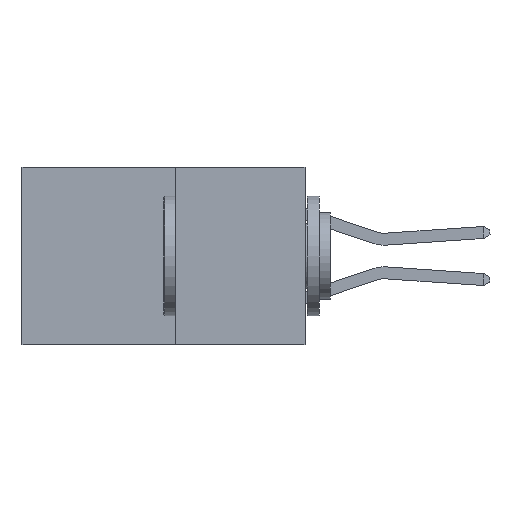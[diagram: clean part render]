
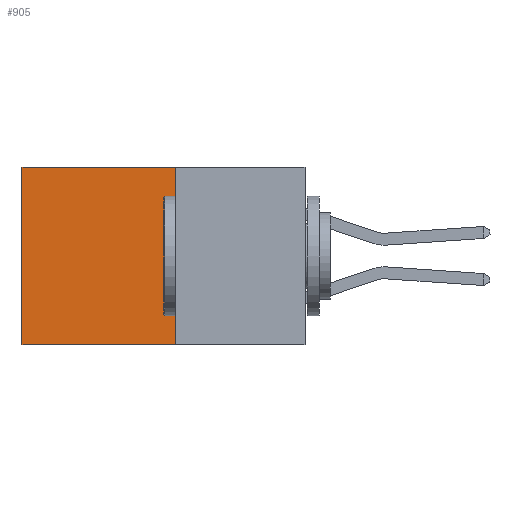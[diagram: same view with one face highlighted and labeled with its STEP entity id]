
A CAD part, left-side view. The second image highlights one B-rep face of the part: STEP entity #905.
In plain terms, the highlighted planar face has unit normal (-1, 0, 0).
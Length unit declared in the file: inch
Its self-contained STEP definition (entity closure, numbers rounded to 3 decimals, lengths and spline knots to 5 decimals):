
#81 = EDGE_CURVE ( 'NONE', #8730, #8609, #4554, .T. ) ;
#905 = ADVANCED_FACE ( 'NONE', ( #2821 ), #7786, .F. ) ;
#1059 = EDGE_CURVE ( 'NONE', #1190, #8609, #7743, .T. ) ;
#1190 = VERTEX_POINT ( 'NONE', #9414 ) ;
#2821 = FACE_OUTER_BOUND ( 'NONE', #2878, .T. ) ;
#2878 = EDGE_LOOP ( 'NONE', ( #4467, #7238, #5087, #5589 ) ) ;
#4222 = AXIS2_PLACEMENT_3D ( 'NONE', #8554, #8684, #8568 ) ;
#4467 = ORIENTED_EDGE ( 'NONE', *, *, #81, .T. ) ;
#4554 = LINE ( 'NONE', #9652, #10314 ) ;
#5087 = ORIENTED_EDGE ( 'NONE', *, *, #10065, .F. ) ;
#5205 = EDGE_CURVE ( 'NONE', #7248, #8730, #9862, .T. ) ;
#5479 = LINE ( 'NONE', #9789, #5730 ) ;
#5589 = ORIENTED_EDGE ( 'NONE', *, *, #5205, .T. ) ;
#5730 = VECTOR ( 'NONE', #10514, 39.37008 ) ;
#5748 = VECTOR ( 'NONE', #8367, 39.37008 ) ;
#5784 = CARTESIAN_POINT ( 'NONE',  ( 0.277, 0.59, -0.37 ) ) ;
#6378 = DIRECTION ( 'NONE',  ( 0., 0., -1. ) ) ;
#7238 = ORIENTED_EDGE ( 'NONE', *, *, #1059, .F. ) ;
#7248 = VERTEX_POINT ( 'NONE', #7903 ) ;
#7373 = CARTESIAN_POINT ( 'NONE',  ( 0.277, 0.59, 0. ) ) ;
#7743 = LINE ( 'NONE', #9202, #5748 ) ;
#7786 = PLANE ( 'NONE',  #4222 ) ;
#7889 = VECTOR ( 'NONE', #9340, 39.37008 ) ;
#7903 = CARTESIAN_POINT ( 'NONE',  ( 0.277, 0.27, 0. ) ) ;
#8367 = DIRECTION ( 'NONE',  ( 0., 1., 0. ) ) ;
#8554 = CARTESIAN_POINT ( 'NONE',  ( 0.277, 0.27, -0.37 ) ) ;
#8568 = DIRECTION ( 'NONE',  ( 0., 0., -1. ) ) ;
#8609 = VERTEX_POINT ( 'NONE', #5784 ) ;
#8684 = DIRECTION ( 'NONE',  ( 1., 0., 0. ) ) ;
#8730 = VERTEX_POINT ( 'NONE', #7373 ) ;
#9202 = CARTESIAN_POINT ( 'NONE',  ( 0.277, 0.27, -0.37 ) ) ;
#9340 = DIRECTION ( 'NONE',  ( 0., 1., 0. ) ) ;
#9393 = CARTESIAN_POINT ( 'NONE',  ( 0.277, 0.27, 0. ) ) ;
#9414 = CARTESIAN_POINT ( 'NONE',  ( 0.277, 0.27, -0.37 ) ) ;
#9652 = CARTESIAN_POINT ( 'NONE',  ( 0.277, 0.59, -0.37 ) ) ;
#9789 = CARTESIAN_POINT ( 'NONE',  ( 0.277, 0.27, -0.37 ) ) ;
#9862 = LINE ( 'NONE', #9393, #7889 ) ;
#10065 = EDGE_CURVE ( 'NONE', #7248, #1190, #5479, .T. ) ;
#10314 = VECTOR ( 'NONE', #6378, 39.37008 ) ;
#10514 = DIRECTION ( 'NONE',  ( 0., 0., -1. ) ) ;
